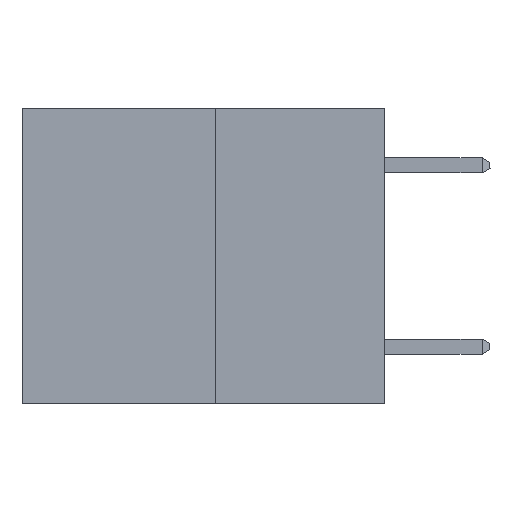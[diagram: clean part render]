
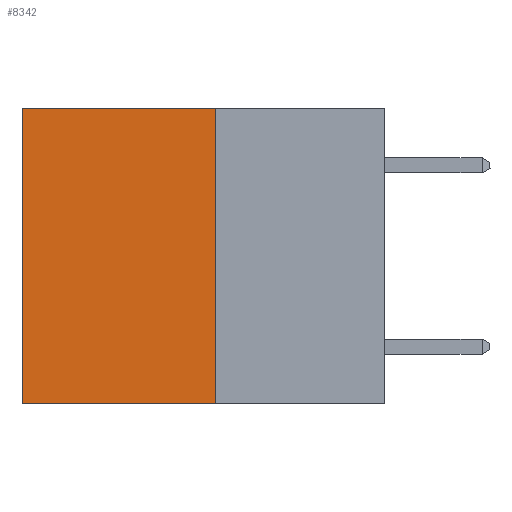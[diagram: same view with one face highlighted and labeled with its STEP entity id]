
A CAD part, left-side view. The second image highlights one B-rep face of the part: STEP entity #8342.
In plain terms, the highlighted planar face has unit normal (-1, 0, 0).
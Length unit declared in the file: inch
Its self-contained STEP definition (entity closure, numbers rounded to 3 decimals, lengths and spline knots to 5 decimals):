
#22 = ORIENTED_EDGE ( 'NONE', *, *, #712, .T. ) ;
#31 = PLANE ( 'NONE',  #14828 ) ;
#712 = EDGE_CURVE ( 'NONE', #2752, #18307, #20542, .T. ) ;
#1066 = ORIENTED_EDGE ( 'NONE', *, *, #20030, .F. ) ;
#1378 = DIRECTION ( 'NONE',  ( 0., 1., 0. ) ) ;
#2060 = ORIENTED_EDGE ( 'NONE', *, *, #19948, .F. ) ;
#2752 = VERTEX_POINT ( 'NONE', #12132 ) ;
#3162 = VECTOR ( 'NONE', #1378, 39.37008 ) ;
#4705 = EDGE_LOOP ( 'NONE', ( #7963, #2060, #1066, #22 ) ) ;
#4752 = CARTESIAN_POINT ( 'NONE',  ( 0.3165, 0.6, -0.49 ) ) ;
#5419 = LINE ( 'NONE', #7121, #17271 ) ;
#7121 = CARTESIAN_POINT ( 'NONE',  ( 0.3165, 0.28, -0.49 ) ) ;
#7242 = CARTESIAN_POINT ( 'NONE',  ( 0.3165, 0.28, -0.49 ) ) ;
#7963 = ORIENTED_EDGE ( 'NONE', *, *, #17599, .T. ) ;
#8342 = ADVANCED_FACE ( 'NONE', ( #20662 ), #31, .F. ) ;
#8368 = CARTESIAN_POINT ( 'NONE',  ( 0.3165, 0.6, -0.49 ) ) ;
#8877 = DIRECTION ( 'NONE',  ( 0., 0., -1. ) ) ;
#10181 = DIRECTION ( 'NONE',  ( 0., 0., -1. ) ) ;
#10657 = CARTESIAN_POINT ( 'NONE',  ( 0.3165, 0.28, -0.49 ) ) ;
#11597 = VECTOR ( 'NONE', #10181, 39.37008 ) ;
#12132 = CARTESIAN_POINT ( 'NONE',  ( 0.3165, 0.28, 0. ) ) ;
#12286 = CARTESIAN_POINT ( 'NONE',  ( 0.3165, 0.28, -0.49 ) ) ;
#14091 = DIRECTION ( 'NONE',  ( 0., 1., 0. ) ) ;
#14542 = DIRECTION ( 'NONE',  ( 1., 0., 0. ) ) ;
#14828 = AXIS2_PLACEMENT_3D ( 'NONE', #7242, #14542, #16375 ) ;
#15252 = LINE ( 'NONE', #12286, #23965 ) ;
#16370 = VERTEX_POINT ( 'NONE', #10657 ) ;
#16375 = DIRECTION ( 'NONE',  ( 0., 0., -1. ) ) ;
#17271 = VECTOR ( 'NONE', #8877, 39.37008 ) ;
#17599 = EDGE_CURVE ( 'NONE', #18307, #17795, #18833, .T. ) ;
#17795 = VERTEX_POINT ( 'NONE', #8368 ) ;
#18307 = VERTEX_POINT ( 'NONE', #22812 ) ;
#18833 = LINE ( 'NONE', #4752, #11597 ) ;
#19948 = EDGE_CURVE ( 'NONE', #16370, #17795, #15252, .T. ) ;
#20030 = EDGE_CURVE ( 'NONE', #2752, #16370, #5419, .T. ) ;
#20542 = LINE ( 'NONE', #20889, #3162 ) ;
#20662 = FACE_OUTER_BOUND ( 'NONE', #4705, .T. ) ;
#20889 = CARTESIAN_POINT ( 'NONE',  ( 0.3165, 0.28, 0. ) ) ;
#22812 = CARTESIAN_POINT ( 'NONE',  ( 0.3165, 0.6, 0. ) ) ;
#23965 = VECTOR ( 'NONE', #14091, 39.37008 ) ;
